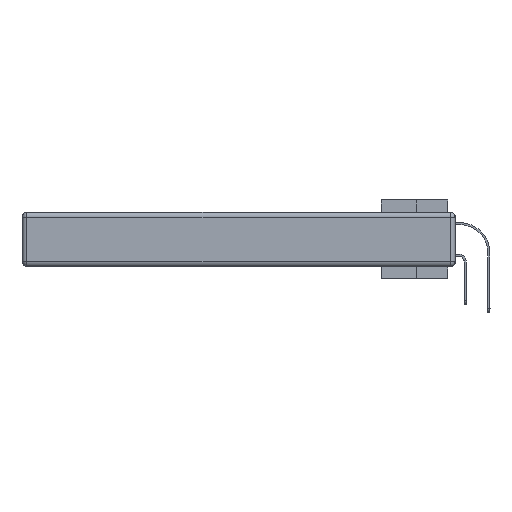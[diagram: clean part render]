
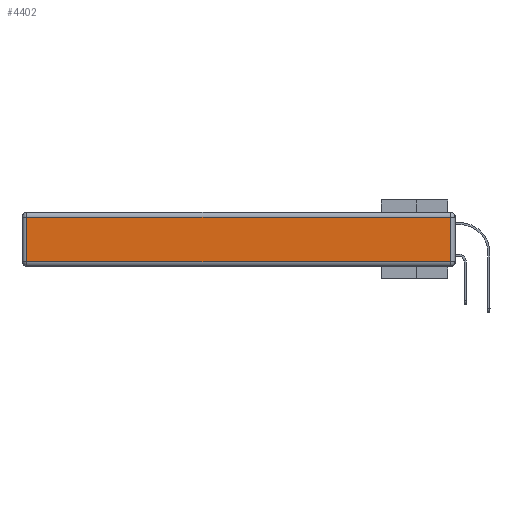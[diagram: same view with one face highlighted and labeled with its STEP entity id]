
A CAD part, left-side view. The second image highlights one B-rep face of the part: STEP entity #4402.
In plain terms, the highlighted planar face has unit normal (-1, 0, 0).
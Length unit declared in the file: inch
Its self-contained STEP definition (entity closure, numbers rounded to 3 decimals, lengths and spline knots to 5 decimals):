
#311 = ORIENTED_EDGE ( 'NONE', *, *, #26079, .T. ) ;
#778 = PLANE ( 'NONE',  #12545 ) ;
#1433 = LINE ( 'NONE', #16866, #24871 ) ;
#1757 = LINE ( 'NONE', #27602, #10864 ) ;
#4402 = ADVANCED_FACE ( 'NONE', ( #13353 ), #778, .T. ) ;
#8475 = LINE ( 'NONE', #30953, #14674 ) ;
#8941 = VERTEX_POINT ( 'NONE', #21010 ) ;
#9318 = DIRECTION ( 'NONE',  ( 0., -1., 0. ) ) ;
#9641 = CARTESIAN_POINT ( 'NONE',  ( 0., 0.03, -0.03 ) ) ;
#10320 = VERTEX_POINT ( 'NONE', #9641 ) ;
#10360 = EDGE_CURVE ( 'NONE', #29047, #10320, #15990, .T. ) ;
#10843 = CARTESIAN_POINT ( 'NONE',  ( 0., 0., -0.343 ) ) ;
#10864 = VECTOR ( 'NONE', #24750, 39.37008 ) ;
#12545 = AXIS2_PLACEMENT_3D ( 'NONE', #10843, #18561, #31468 ) ;
#13353 = FACE_OUTER_BOUND ( 'NONE', #16431, .T. ) ;
#14239 = ORIENTED_EDGE ( 'NONE', *, *, #10360, .T. ) ;
#14674 = VECTOR ( 'NONE', #15858, 39.37008 ) ;
#14712 = EDGE_CURVE ( 'NONE', #10320, #8941, #8475, .T. ) ;
#15858 = DIRECTION ( 'NONE',  ( 0., 1., 0. ) ) ;
#15990 = LINE ( 'NONE', #25726, #24497 ) ;
#16431 = EDGE_LOOP ( 'NONE', ( #17431, #14239, #16699, #311 ) ) ;
#16699 = ORIENTED_EDGE ( 'NONE', *, *, #14712, .T. ) ;
#16866 = CARTESIAN_POINT ( 'NONE',  ( 0., 0., -0.313 ) ) ;
#17431 = ORIENTED_EDGE ( 'NONE', *, *, #21328, .T. ) ;
#18561 = DIRECTION ( 'NONE',  ( -1., 0., 0. ) ) ;
#21010 = CARTESIAN_POINT ( 'NONE',  ( 0., 2.72, -0.03 ) ) ;
#21328 = EDGE_CURVE ( 'NONE', #28868, #29047, #1433, .T. ) ;
#23542 = DIRECTION ( 'NONE',  ( 0., 0., 1. ) ) ;
#24211 = CARTESIAN_POINT ( 'NONE',  ( 0., 0.03, -0.313 ) ) ;
#24497 = VECTOR ( 'NONE', #23542, 39.37008 ) ;
#24750 = DIRECTION ( 'NONE',  ( 0., 0., -1. ) ) ;
#24871 = VECTOR ( 'NONE', #9318, 39.37008 ) ;
#25726 = CARTESIAN_POINT ( 'NONE',  ( 0., 0.03, -0.343 ) ) ;
#26079 = EDGE_CURVE ( 'NONE', #8941, #28868, #1757, .T. ) ;
#27602 = CARTESIAN_POINT ( 'NONE',  ( 0., 2.72, -0.343 ) ) ;
#27920 = CARTESIAN_POINT ( 'NONE',  ( 0., 2.72, -0.313 ) ) ;
#28868 = VERTEX_POINT ( 'NONE', #27920 ) ;
#29047 = VERTEX_POINT ( 'NONE', #24211 ) ;
#30953 = CARTESIAN_POINT ( 'NONE',  ( 0., 2.75, -0.03 ) ) ;
#31468 = DIRECTION ( 'NONE',  ( 0., 0., 1. ) ) ;
